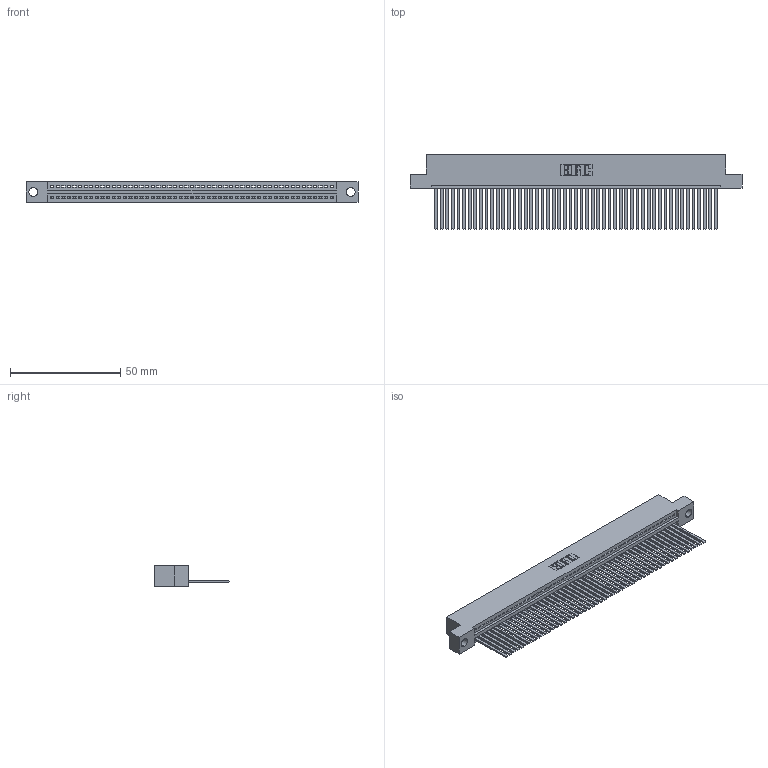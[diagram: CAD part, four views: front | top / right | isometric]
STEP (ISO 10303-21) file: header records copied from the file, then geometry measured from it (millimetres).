
FILE_DESCRIPTION (( 'STEP AP203' ), '1' );
FILE_NAME ('345-051-544-104.STEP', '2018-09-22T18:13:43', ( '' ), ( '' ), 'SwSTEP 2.0', 'SolidWorks 2016', '' );
FILE_SCHEMA (( 'CONFIG_CONTROL_DESIGN' ));
Length unit declared in the file: inch
Products named in the file (3): 345 Part_Flush Mounting Lugs - 0.156 Dia-TH; 345-292-001_345-293-144; 345-051-544-104
Assembly tree (52 placements, depth 2):
  345-051-544-104
    345 Part_Flush Mounting Lugs - 0.156 Dia-TH
    345-292-001_345-293-144  x51
Bounding box: 150.75 x 33.96 x 9.4 mm (x, y, z)
Volume: 14894.8 mm3; surface area: 21498.1 mm2
Topology: 52 solids, 52 shells, 2778 faces, 8399 edges, 5530 vertices
Faces by surface type: plane 1916, cylinder 862
Entity records: 36991 total; most frequent: CARTESIAN_POINT 6413, ORIENTED_EDGE 6398, DIRECTION 5585, EDGE_CURVE 3199, LINE 2867, VECTOR 2867, VERTEX_POINT 2130, AXIS2_PLACEMENT_3D 1359
